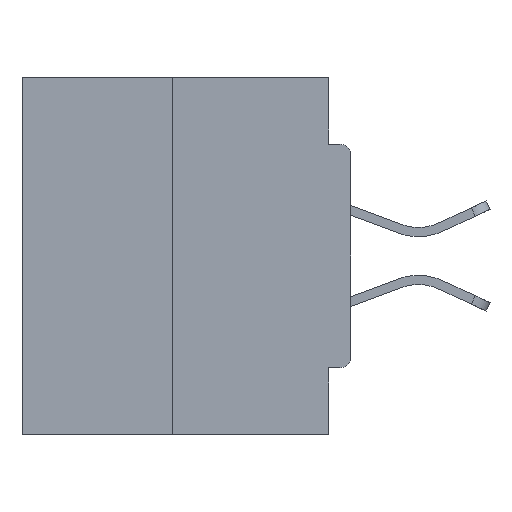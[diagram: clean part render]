
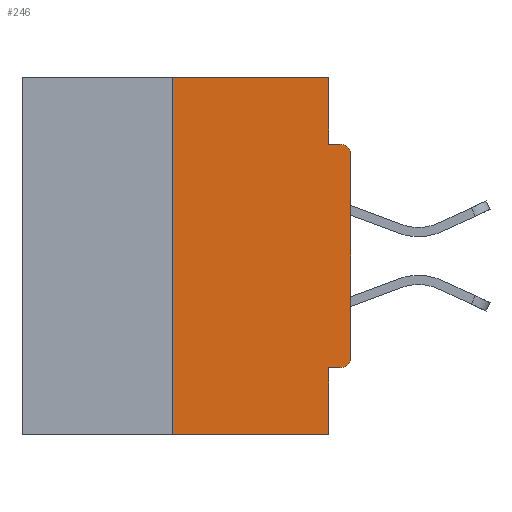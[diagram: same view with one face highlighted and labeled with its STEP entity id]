
A CAD part, left-side view. The second image highlights one B-rep face of the part: STEP entity #246.
In plain terms, the highlighted planar face has unit normal (-1, 0, 0).
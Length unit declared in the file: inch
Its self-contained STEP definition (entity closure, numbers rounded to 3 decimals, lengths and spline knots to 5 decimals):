
#246 = ADVANCED_FACE ( 'NONE', ( #6035 ), #19157, .F. ) ;
#1051 = CARTESIAN_POINT ( 'NONE',  ( 0., 0., -0.4065 ) ) ;
#1109 = CARTESIAN_POINT ( 'NONE',  ( 0., 0., -0.0935 ) ) ;
#1433 = CARTESIAN_POINT ( 'NONE',  ( 0., 0.031, -0.5 ) ) ;
#1634 = EDGE_CURVE ( 'NONE', #24000, #21194, #28078, .T. ) ;
#1804 = CARTESIAN_POINT ( 'NONE',  ( 0., 0., -0.3915 ) ) ;
#2233 = CARTESIAN_POINT ( 'NONE',  ( 0., 0.46, -0.5 ) ) ;
#3868 = LINE ( 'NONE', #1051, #9292 ) ;
#4884 = ORIENTED_EDGE ( 'NONE', *, *, #26551, .T. ) ;
#5398 = CARTESIAN_POINT ( 'NONE',  ( 0., 0.015, -0.3915 ) ) ;
#5853 = CARTESIAN_POINT ( 'NONE',  ( 0., 0.46, 0. ) ) ;
#6035 = FACE_OUTER_BOUND ( 'NONE', #23209, .T. ) ;
#6064 = VERTEX_POINT ( 'NONE', #8996 ) ;
#6751 = CARTESIAN_POINT ( 'NONE',  ( 0., 0.031, 0. ) ) ;
#7166 = VECTOR ( 'NONE', #20649, 39.37008 ) ;
#7510 = VECTOR ( 'NONE', #10628, 39.37008 ) ;
#8301 = EDGE_CURVE ( 'NONE', #6064, #21430, #12158, .T. ) ;
#8477 = CARTESIAN_POINT ( 'NONE',  ( 0., 0.015, -0.1085 ) ) ;
#8665 = DIRECTION ( 'NONE',  ( 0., 1., 0. ) ) ;
#8753 = DIRECTION ( 'NONE',  ( 0., 0., -1. ) ) ;
#8996 = CARTESIAN_POINT ( 'NONE',  ( 0., 0.031, -0.4065 ) ) ;
#9274 = EDGE_CURVE ( 'NONE', #33968, #21430, #10818, .T. ) ;
#9292 = VECTOR ( 'NONE', #8665, 39.37008 ) ;
#9525 = DIRECTION ( 'NONE',  ( 0., -1., 0. ) ) ;
#10628 = DIRECTION ( 'NONE',  ( 0., -1., 0. ) ) ;
#10818 = LINE ( 'NONE', #2233, #7510 ) ;
#11035 = CIRCLE ( 'NONE', #22684, 0.015 ) ;
#11610 = CARTESIAN_POINT ( 'NONE',  ( 0., 0.25, -0.5 ) ) ;
#12158 = LINE ( 'NONE', #1433, #15928 ) ;
#12262 = DIRECTION ( 'NONE',  ( 0., 0., 1. ) ) ;
#12647 = CARTESIAN_POINT ( 'NONE',  ( 0., 0.031, 0. ) ) ;
#13032 = VERTEX_POINT ( 'NONE', #1804 ) ;
#13174 = CARTESIAN_POINT ( 'NONE',  ( 0., 0.25, 0. ) ) ;
#13302 = ORIENTED_EDGE ( 'NONE', *, *, #32942, .T. ) ;
#14256 = VERTEX_POINT ( 'NONE', #28379 ) ;
#14288 = ORIENTED_EDGE ( 'NONE', *, *, #24867, .F. ) ;
#14491 = VECTOR ( 'NONE', #20957, 39.37008 ) ;
#15734 = LINE ( 'NONE', #34241, #14491 ) ;
#15928 = VECTOR ( 'NONE', #25331, 39.37008 ) ;
#16033 = VECTOR ( 'NONE', #12262, 39.37008 ) ;
#16157 = DIRECTION ( 'NONE',  ( -1., 0., 0. ) ) ;
#16933 = AXIS2_PLACEMENT_3D ( 'NONE', #8477, #16157, #29818 ) ;
#17932 = CIRCLE ( 'NONE', #16933, 0.015 ) ;
#18003 = VECTOR ( 'NONE', #27523, 39.37008 ) ;
#18353 = DIRECTION ( 'NONE',  ( -1., 0., 0. ) ) ;
#19157 = PLANE ( 'NONE',  #27280 ) ;
#19691 = ORIENTED_EDGE ( 'NONE', *, *, #8301, .F. ) ;
#19783 = CARTESIAN_POINT ( 'NONE',  ( 0., 0., 0. ) ) ;
#19836 = ORIENTED_EDGE ( 'NONE', *, *, #1634, .F. ) ;
#19952 = EDGE_CURVE ( 'NONE', #13032, #14256, #22371, .T. ) ;
#20649 = DIRECTION ( 'NONE',  ( 0., 0., -1. ) ) ;
#20957 = DIRECTION ( 'NONE',  ( 0., 0., 1. ) ) ;
#21194 = VERTEX_POINT ( 'NONE', #6751 ) ;
#21430 = VERTEX_POINT ( 'NONE', #24815 ) ;
#22167 = ORIENTED_EDGE ( 'NONE', *, *, #22311, .F. ) ;
#22208 = DIRECTION ( 'NONE',  ( 1., 0., 0. ) ) ;
#22311 = EDGE_CURVE ( 'NONE', #27560, #26614, #32215, .T. ) ;
#22371 = LINE ( 'NONE', #19783, #16033 ) ;
#22590 = ORIENTED_EDGE ( 'NONE', *, *, #19952, .T. ) ;
#22684 = AXIS2_PLACEMENT_3D ( 'NONE', #5398, #18353, #26665 ) ;
#23034 = CARTESIAN_POINT ( 'NONE',  ( 0., 0.031, -0.0935 ) ) ;
#23045 = ORIENTED_EDGE ( 'NONE', *, *, #9274, .T. ) ;
#23209 = EDGE_LOOP ( 'NONE', ( #19836, #30443, #23045, #19691, #27570, #13302, #22590, #4884, #22167, #14288 ) ) ;
#24000 = VERTEX_POINT ( 'NONE', #13174 ) ;
#24815 = CARTESIAN_POINT ( 'NONE',  ( 0., 0.031, -0.5 ) ) ;
#24867 = EDGE_CURVE ( 'NONE', #21194, #27560, #32206, .T. ) ;
#25331 = DIRECTION ( 'NONE',  ( 0., 0., -1. ) ) ;
#25593 = CARTESIAN_POINT ( 'NONE',  ( 0., 0.46, 0. ) ) ;
#25622 = VECTOR ( 'NONE', #9525, 39.37008 ) ;
#26551 = EDGE_CURVE ( 'NONE', #14256, #26614, #17932, .T. ) ;
#26614 = VERTEX_POINT ( 'NONE', #30286 ) ;
#26665 = DIRECTION ( 'NONE',  ( 0., 0., -1. ) ) ;
#27280 = AXIS2_PLACEMENT_3D ( 'NONE', #5853, #22208, #8753 ) ;
#27523 = DIRECTION ( 'NONE',  ( 0., -1., 0. ) ) ;
#27532 = EDGE_CURVE ( 'NONE', #33968, #24000, #15734, .T. ) ;
#27560 = VERTEX_POINT ( 'NONE', #23034 ) ;
#27570 = ORIENTED_EDGE ( 'NONE', *, *, #30339, .F. ) ;
#28078 = LINE ( 'NONE', #25593, #25622 ) ;
#28379 = CARTESIAN_POINT ( 'NONE',  ( 0., 0., -0.1085 ) ) ;
#29818 = DIRECTION ( 'NONE',  ( 0., 0., -1. ) ) ;
#30184 = CARTESIAN_POINT ( 'NONE',  ( 0., 0.015, -0.4065 ) ) ;
#30286 = CARTESIAN_POINT ( 'NONE',  ( 0., 0.015, -0.0935 ) ) ;
#30339 = EDGE_CURVE ( 'NONE', #32346, #6064, #3868, .T. ) ;
#30443 = ORIENTED_EDGE ( 'NONE', *, *, #27532, .F. ) ;
#32206 = LINE ( 'NONE', #12647, #7166 ) ;
#32215 = LINE ( 'NONE', #1109, #18003 ) ;
#32346 = VERTEX_POINT ( 'NONE', #30184 ) ;
#32942 = EDGE_CURVE ( 'NONE', #32346, #13032, #11035, .T. ) ;
#33968 = VERTEX_POINT ( 'NONE', #11610 ) ;
#34241 = CARTESIAN_POINT ( 'NONE',  ( 0., 0.25, 0. ) ) ;
